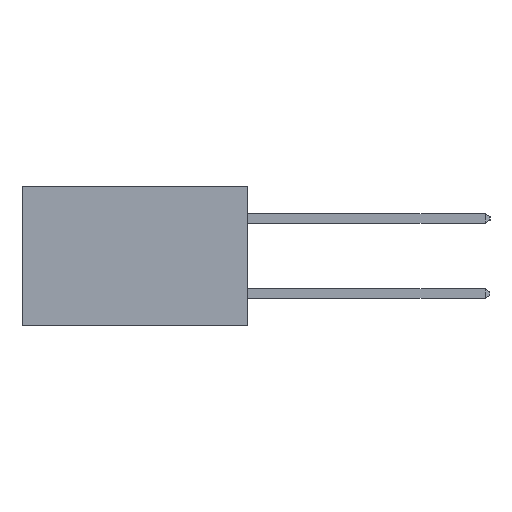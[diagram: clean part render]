
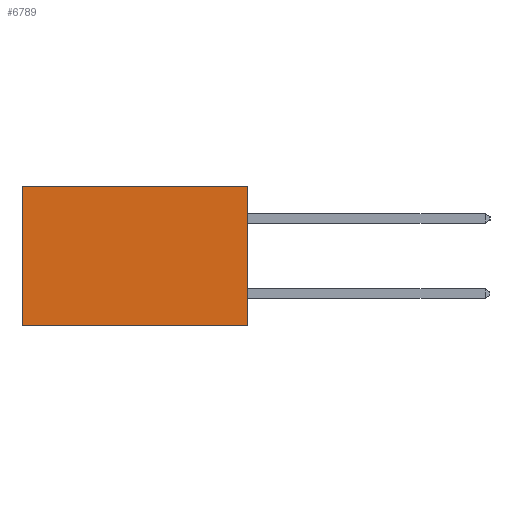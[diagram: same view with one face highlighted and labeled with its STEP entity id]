
A CAD part, left-side view. The second image highlights one B-rep face of the part: STEP entity #6789.
In plain terms, the highlighted planar face has unit normal (-1, 0, 0).
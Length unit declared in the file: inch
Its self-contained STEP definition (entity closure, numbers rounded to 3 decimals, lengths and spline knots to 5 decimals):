
#509 = CARTESIAN_POINT ( 'NONE',  ( 0.298, 0., -0.37 ) ) ;
#775 = DIRECTION ( 'NONE',  ( 0., 0., -1. ) ) ;
#796 = DIRECTION ( 'NONE',  ( 1., 0., 0. ) ) ;
#837 = PLANE ( 'NONE',  #11326 ) ;
#1118 = CARTESIAN_POINT ( 'NONE',  ( 0.298, 0., 0. ) ) ;
#2687 = LINE ( 'NONE', #3620, #6423 ) ;
#3505 = VERTEX_POINT ( 'NONE', #9858 ) ;
#3620 = CARTESIAN_POINT ( 'NONE',  ( 0.298, 0.6, 0. ) ) ;
#3660 = LINE ( 'NONE', #9901, #17412 ) ;
#5210 = EDGE_CURVE ( 'NONE', #3505, #15023, #12830, .T. ) ;
#5646 = VERTEX_POINT ( 'NONE', #15506 ) ;
#5904 = EDGE_CURVE ( 'NONE', #8408, #5646, #9476, .T. ) ;
#6011 = DIRECTION ( 'NONE',  ( 0., 0., -1. ) ) ;
#6423 = VECTOR ( 'NONE', #6011, 39.37008 ) ;
#6563 = EDGE_CURVE ( 'NONE', #3505, #8408, #3660, .T. ) ;
#6728 = ORIENTED_EDGE ( 'NONE', *, *, #5210, .T. ) ;
#6789 = ADVANCED_FACE ( 'NONE', ( #11736 ), #837, .F. ) ;
#6881 = EDGE_CURVE ( 'NONE', #15023, #5646, #2687, .T. ) ;
#7567 = ORIENTED_EDGE ( 'NONE', *, *, #6563, .F. ) ;
#7874 = CARTESIAN_POINT ( 'NONE',  ( 0.298, 0., 0. ) ) ;
#8408 = VERTEX_POINT ( 'NONE', #12825 ) ;
#9476 = LINE ( 'NONE', #509, #12150 ) ;
#9479 = DIRECTION ( 'NONE',  ( 0., 1., 0. ) ) ;
#9858 = CARTESIAN_POINT ( 'NONE',  ( 0.298, 0., 0. ) ) ;
#9901 = CARTESIAN_POINT ( 'NONE',  ( 0.298, 0., 0. ) ) ;
#10824 = EDGE_LOOP ( 'NONE', ( #12457, #11693, #7567, #6728 ) ) ;
#10826 = DIRECTION ( 'NONE',  ( 0., 1., 0. ) ) ;
#11326 = AXIS2_PLACEMENT_3D ( 'NONE', #1118, #796, #775 ) ;
#11693 = ORIENTED_EDGE ( 'NONE', *, *, #5904, .F. ) ;
#11736 = FACE_OUTER_BOUND ( 'NONE', #10824, .T. ) ;
#12150 = VECTOR ( 'NONE', #10826, 39.37008 ) ;
#12261 = DIRECTION ( 'NONE',  ( 0., 0., -1. ) ) ;
#12457 = ORIENTED_EDGE ( 'NONE', *, *, #6881, .T. ) ;
#12825 = CARTESIAN_POINT ( 'NONE',  ( 0.298, 0., -0.37 ) ) ;
#12830 = LINE ( 'NONE', #7874, #16548 ) ;
#15023 = VERTEX_POINT ( 'NONE', #17099 ) ;
#15506 = CARTESIAN_POINT ( 'NONE',  ( 0.298, 0.6, -0.37 ) ) ;
#16548 = VECTOR ( 'NONE', #9479, 39.37008 ) ;
#17099 = CARTESIAN_POINT ( 'NONE',  ( 0.298, 0.6, 0. ) ) ;
#17412 = VECTOR ( 'NONE', #12261, 39.37008 ) ;
